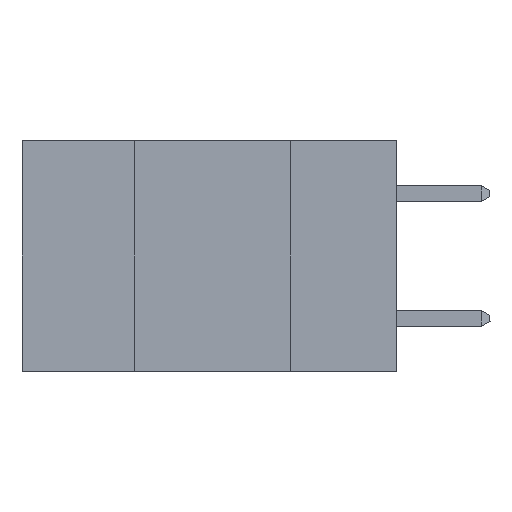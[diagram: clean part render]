
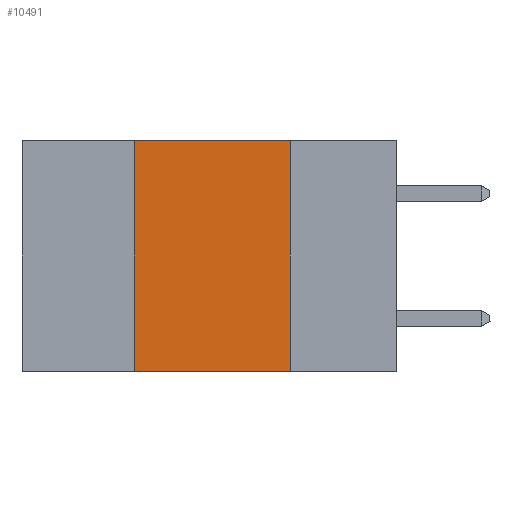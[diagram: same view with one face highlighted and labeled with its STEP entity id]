
A CAD part, left-side view. The second image highlights one B-rep face of the part: STEP entity #10491.
In plain terms, the highlighted planar face has unit normal (-1, 0, 0).
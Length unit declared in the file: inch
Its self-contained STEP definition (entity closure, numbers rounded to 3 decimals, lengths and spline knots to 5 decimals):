
#121 = DIRECTION ( 'NONE',  ( 0., 0., -1. ) ) ;
#220 = FACE_OUTER_BOUND ( 'NONE', #11960, .T. ) ;
#2523 = CARTESIAN_POINT ( 'NONE',  ( 0., 0.42, -0.37 ) ) ;
#3373 = ORIENTED_EDGE ( 'NONE', *, *, #23249, .F. ) ;
#3436 = LINE ( 'NONE', #4619, #26919 ) ;
#3763 = VERTEX_POINT ( 'NONE', #14718 ) ;
#4234 = VERTEX_POINT ( 'NONE', #2523 ) ;
#4562 = PLANE ( 'NONE',  #24016 ) ;
#4619 = CARTESIAN_POINT ( 'NONE',  ( 0., 0.17, 0. ) ) ;
#6188 = CARTESIAN_POINT ( 'NONE',  ( 0., 0.6, -0.37 ) ) ;
#6888 = CARTESIAN_POINT ( 'NONE',  ( 0., 0.6, 0. ) ) ;
#8519 = DIRECTION ( 'NONE',  ( 0., -1., 0. ) ) ;
#9222 = DIRECTION ( 'NONE',  ( 1., 0., 0. ) ) ;
#10433 = LINE ( 'NONE', #29241, #21075 ) ;
#10491 = ADVANCED_FACE ( 'NONE', ( #220 ), #4562, .F. ) ;
#11669 = VECTOR ( 'NONE', #13922, 39.37008 ) ;
#11960 = EDGE_LOOP ( 'NONE', ( #24731, #27578, #3373, #15268 ) ) ;
#12786 = CARTESIAN_POINT ( 'NONE',  ( 0., 0.42, 0. ) ) ;
#13922 = DIRECTION ( 'NONE',  ( 0., 0., 1. ) ) ;
#14718 = CARTESIAN_POINT ( 'NONE',  ( 0., 0.17, 0. ) ) ;
#15268 = ORIENTED_EDGE ( 'NONE', *, *, #15531, .T. ) ;
#15531 = EDGE_CURVE ( 'NONE', #4234, #21119, #28382, .T. ) ;
#16461 = VECTOR ( 'NONE', #8519, 39.37008 ) ;
#16477 = EDGE_CURVE ( 'NONE', #3763, #21119, #3436, .T. ) ;
#18121 = DIRECTION ( 'NONE',  ( 0., -1., 0. ) ) ;
#19026 = VERTEX_POINT ( 'NONE', #12786 ) ;
#21075 = VECTOR ( 'NONE', #18121, 39.37008 ) ;
#21119 = VERTEX_POINT ( 'NONE', #25020 ) ;
#23249 = EDGE_CURVE ( 'NONE', #4234, #19026, #23696, .T. ) ;
#23696 = LINE ( 'NONE', #27512, #11669 ) ;
#24016 = AXIS2_PLACEMENT_3D ( 'NONE', #6888, #9222, #25043 ) ;
#24731 = ORIENTED_EDGE ( 'NONE', *, *, #16477, .F. ) ;
#25020 = CARTESIAN_POINT ( 'NONE',  ( 0., 0.17, -0.37 ) ) ;
#25043 = DIRECTION ( 'NONE',  ( 0., 0., -1. ) ) ;
#25694 = EDGE_CURVE ( 'NONE', #19026, #3763, #10433, .T. ) ;
#26919 = VECTOR ( 'NONE', #121, 39.37008 ) ;
#27512 = CARTESIAN_POINT ( 'NONE',  ( 0., 0.42, 0. ) ) ;
#27578 = ORIENTED_EDGE ( 'NONE', *, *, #25694, .F. ) ;
#28382 = LINE ( 'NONE', #6188, #16461 ) ;
#29241 = CARTESIAN_POINT ( 'NONE',  ( 0., 0.6, 0. ) ) ;
